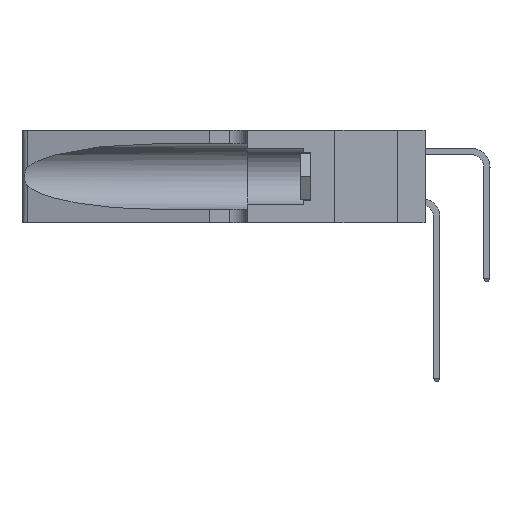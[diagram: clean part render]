
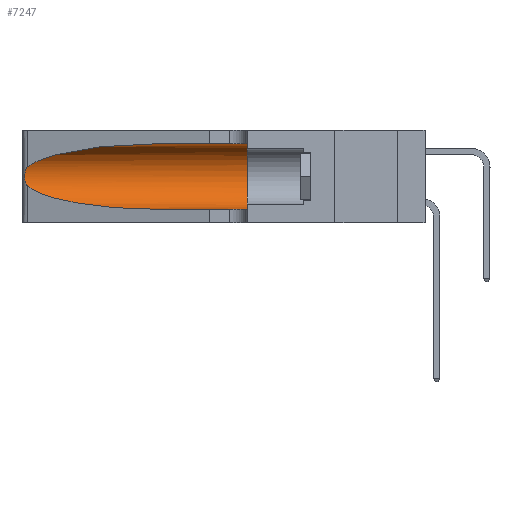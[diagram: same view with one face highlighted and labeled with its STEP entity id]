
A CAD part, left-side view. The second image highlights one B-rep face of the part: STEP entity #7247.
In plain terms, the highlighted cylindrical face has radius 3.308 mm (diameter 6.617 mm), a partial arc.
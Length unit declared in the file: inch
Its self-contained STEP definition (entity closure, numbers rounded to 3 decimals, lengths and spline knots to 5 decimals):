
#1663 = DIRECTION ( 'NONE',  ( 0., -1., 0. ) ) ;
#3095 = CARTESIAN_POINT ( 'NONE',  ( 0.25787, 1.23484, 0.2124 ) ) ;
#3348 = CIRCLE ( 'NONE', #35188, 0.13025 ) ;
#4124 = DIRECTION ( 'NONE',  ( 0., -1., 0. ) ) ;
#4462 = CARTESIAN_POINT ( 'NONE',  ( 0.1305, 0.35, 0.31525 ) ) ;
#5332 =( BOUNDED_CURVE ( )  B_SPLINE_CURVE ( 3, ( #31411, #10853, #13824, #34363 ),
 .UNSPECIFIED., .F., .T. ) 
 B_SPLINE_CURVE_WITH_KNOTS ( ( 4, 4 ),
 ( 1.5708, 2.84003 ),
 .UNSPECIFIED. ) 
 CURVE ( )  GEOMETRIC_REPRESENTATION_ITEM ( )  RATIONAL_B_SPLINE_CURVE ( ( 1., 0.87, 0.87, 1. ) ) 
 REPRESENTATION_ITEM ( '' )  );
#6072 = CARTESIAN_POINT ( 'NONE',  ( 0.26018, 1.23835, 0.19895 ) ) ;
#6582 = DIRECTION ( 'NONE',  ( 0., 0., -1. ) ) ;
#7147 = CARTESIAN_POINT ( 'NONE',  ( 0.1305, 1.61858, 0.05475 ) ) ;
#7247 = ADVANCED_FACE ( 'NONE', ( #34910 ), #19292, .F. ) ;
#7613 = CARTESIAN_POINT ( 'NONE',  ( 0.1305, 0.72297, 0.31525 ) ) ;
#7616 = EDGE_CURVE ( 'NONE', #28840, #8911, #16568, .T. ) ;
#7651 = DIRECTION ( 'NONE',  ( 0., 1., 0. ) ) ;
#8452 = EDGE_CURVE ( 'NONE', #19560, #34160, #5332, .T. ) ;
#8911 = VERTEX_POINT ( 'NONE', #27541 ) ;
#9138 = CARTESIAN_POINT ( 'NONE',  ( 0.26075, 1.23896, 0.178 ) ) ;
#9230 = ORIENTED_EDGE ( 'NONE', *, *, #24325, .F. ) ;
#9830 = AXIS2_PLACEMENT_3D ( 'NONE', #27218, #24270, #6582 ) ;
#10020 = CARTESIAN_POINT ( 'NONE',  ( 0.18966, 0.96281, 0.05475 ) ) ;
#10853 = CARTESIAN_POINT ( 'NONE',  ( 0.18966, 0.96281, 0.31525 ) ) ;
#12056 = CARTESIAN_POINT ( 'NONE',  ( 0.25856, 1.23593, 0.16098 ) ) ;
#13824 = CARTESIAN_POINT ( 'NONE',  ( 0.2373, 1.15595, 0.28018 ) ) ;
#14115 = CARTESIAN_POINT ( 'NONE',  ( 0.1305, 0.72297, 0.05475 ) ) ;
#14294 = VERTEX_POINT ( 'NONE', #24235 ) ;
#14323 = VERTEX_POINT ( 'NONE', #4462 ) ;
#15037 = CARTESIAN_POINT ( 'NONE',  ( 0.25639, 1.23186, 0.15144 ) ) ;
#16257 = B_SPLINE_CURVE_WITH_KNOTS ( 'NONE', 3,
 ( #17855, #35442, #20807, #3095, #23799, #6072, #26728, #9138, #29693, #12056, #32627, #15037, #35572, #17979 ),
 .UNSPECIFIED., .F., .F.,
 ( 4, 2, 2, 2, 2, 2, 4 ),
 ( 0., 0.00027, 0.00053, 0.00107, 0.0016, 0.00187, 0.00214 ),
 .UNSPECIFIED. ) ;
#16531 = ORIENTED_EDGE ( 'NONE', *, *, #36740, .T. ) ;
#16568 = LINE ( 'NONE', #7147, #38149 ) ;
#17855 = CARTESIAN_POINT ( 'NONE',  ( 0.25487, 1.22718, 0.22369 ) ) ;
#17891 = VECTOR ( 'NONE', #1663, 39.37008 ) ;
#17979 = CARTESIAN_POINT ( 'NONE',  ( 0.25487, 1.22718, 0.14631 ) ) ;
#18576 = EDGE_CURVE ( 'NONE', #34160, #14294, #16257, .T. ) ;
#19292 = CYLINDRICAL_SURFACE ( 'NONE', #9830, 0.13025 ) ;
#19560 = VERTEX_POINT ( 'NONE', #7613 ) ;
#19953 = CARTESIAN_POINT ( 'NONE',  ( 0.25487, 1.22718, 0.22369 ) ) ;
#20213 = ORIENTED_EDGE ( 'NONE', *, *, #7616, .T. ) ;
#20807 = CARTESIAN_POINT ( 'NONE',  ( 0.25639, 1.23184, 0.21858 ) ) ;
#23524 = ORIENTED_EDGE ( 'NONE', *, *, #18576, .T. ) ;
#23799 = CARTESIAN_POINT ( 'NONE',  ( 0.25854, 1.2359, 0.20912 ) ) ;
#24235 = CARTESIAN_POINT ( 'NONE',  ( 0.25487, 1.22718, 0.14631 ) ) ;
#24270 = DIRECTION ( 'NONE',  ( 0., -1., 0. ) ) ;
#24325 = EDGE_CURVE ( 'NONE', #14323, #8911, #3348, .T. ) ;
#24671 = CARTESIAN_POINT ( 'NONE',  ( 0.25487, 1.22718, 0.14631 ) ) ;
#25291 = CARTESIAN_POINT ( 'NONE',  ( 0.1305, 0.35, 0.185 ) ) ;
#25614 = EDGE_LOOP ( 'NONE', ( #35001, #23524, #16531, #20213, #9230, #26127 ) ) ;
#25743 = LINE ( 'NONE', #37010, #17891 ) ;
#26127 = ORIENTED_EDGE ( 'NONE', *, *, #30052, .F. ) ;
#26728 = CARTESIAN_POINT ( 'NONE',  ( 0.26075, 1.23896, 0.19203 ) ) ;
#27218 = CARTESIAN_POINT ( 'NONE',  ( 0.1305, 1.61858, 0.185 ) ) ;
#27541 = CARTESIAN_POINT ( 'NONE',  ( 0.1305, 0.35, 0.05475 ) ) ;
#27624 = CARTESIAN_POINT ( 'NONE',  ( 0.2373, 1.15595, 0.08982 ) ) ;
#28261 = DIRECTION ( 'NONE',  ( 0., 0., 1. ) ) ;
#28840 = VERTEX_POINT ( 'NONE', #14115 ) ;
#29693 = CARTESIAN_POINT ( 'NONE',  ( 0.26017, 1.23833, 0.17102 ) ) ;
#30052 = EDGE_CURVE ( 'NONE', #19560, #14323, #25743, .T. ) ;
#30573 = CARTESIAN_POINT ( 'NONE',  ( 0.1305, 0.72297, 0.05475 ) ) ;
#31411 = CARTESIAN_POINT ( 'NONE',  ( 0.1305, 0.72297, 0.31525 ) ) ;
#32627 = CARTESIAN_POINT ( 'NONE',  ( 0.25789, 1.23486, 0.15765 ) ) ;
#34160 = VERTEX_POINT ( 'NONE', #19953 ) ;
#34363 = CARTESIAN_POINT ( 'NONE',  ( 0.25487, 1.22718, 0.22369 ) ) ;
#34910 = FACE_OUTER_BOUND ( 'NONE', #25614, .T. ) ;
#35001 = ORIENTED_EDGE ( 'NONE', *, *, #8452, .T. ) ;
#35188 = AXIS2_PLACEMENT_3D ( 'NONE', #25291, #7651, #28261 ) ;
#35442 = CARTESIAN_POINT ( 'NONE',  ( 0.25555, 1.22994, 0.2215 ) ) ;
#35572 = CARTESIAN_POINT ( 'NONE',  ( 0.25555, 1.22993, 0.14849 ) ) ;
#36740 = EDGE_CURVE ( 'NONE', #14294, #28840, #37919, .T. ) ;
#37010 = CARTESIAN_POINT ( 'NONE',  ( 0.1305, 1.61858, 0.31525 ) ) ;
#37919 =( BOUNDED_CURVE ( )  B_SPLINE_CURVE ( 3, ( #24671, #27624, #10020, #30573 ),
 .UNSPECIFIED., .F., .T. ) 
 B_SPLINE_CURVE_WITH_KNOTS ( ( 4, 4 ),
 ( 3.44316, 4.71239 ),
 .UNSPECIFIED. ) 
 CURVE ( )  GEOMETRIC_REPRESENTATION_ITEM ( )  RATIONAL_B_SPLINE_CURVE ( ( 1., 0.87, 0.87, 1. ) ) 
 REPRESENTATION_ITEM ( '' )  );
#38149 = VECTOR ( 'NONE', #4124, 39.37008 ) ;
